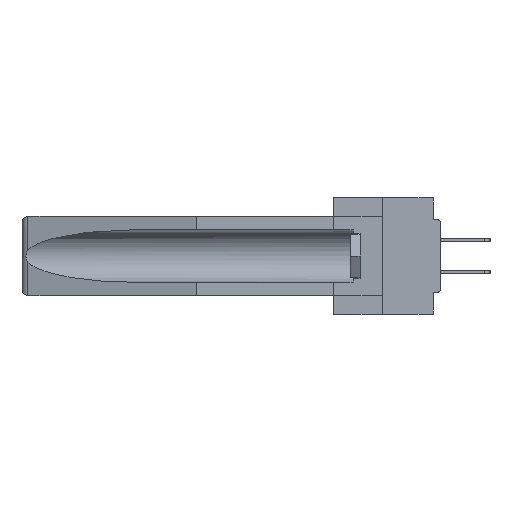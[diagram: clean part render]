
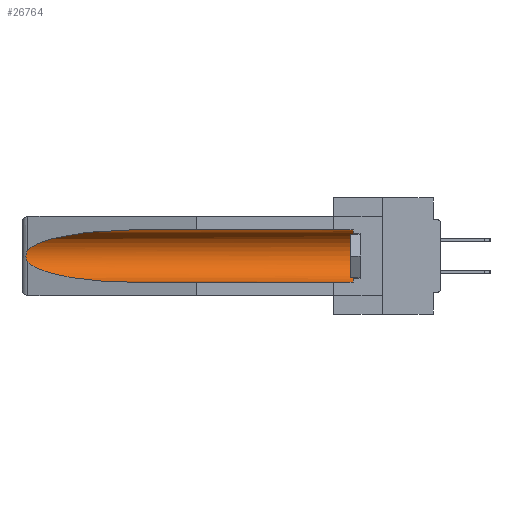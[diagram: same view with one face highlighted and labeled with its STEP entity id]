
A CAD part, left-side view. The second image highlights one B-rep face of the part: STEP entity #26764.
In plain terms, the highlighted cylindrical face has radius 2.857 mm (diameter 5.715 mm), a partial arc.
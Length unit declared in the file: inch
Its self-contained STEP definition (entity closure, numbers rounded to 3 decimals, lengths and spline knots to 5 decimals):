
#1391 = DIRECTION ( 'NONE',  ( 0., -1., 0. ) ) ;
#2315 = CARTESIAN_POINT ( 'NONE',  ( 0.26537, 1.52718, -0.14972 ) ) ;
#2496 = CARTESIAN_POINT ( 'NONE',  ( 0.155, 1.07973, -0.284 ) ) ;
#2711 = CARTESIAN_POINT ( 'NONE',  ( 0.26655, 1.53094, -0.18657 ) ) ;
#2994 = CARTESIAN_POINT ( 'NONE',  ( 0.155, -0.30754, -0.284 ) ) ;
#4425 = ORIENTED_EDGE ( 'NONE', *, *, #5742, .T. ) ;
#5557 = CARTESIAN_POINT ( 'NONE',  ( 0.155, -0.30754, -0.059 ) ) ;
#5742 = EDGE_CURVE ( 'NONE', #29411, #37404, #18426, .T. ) ;
#5941 = AXIS2_PLACEMENT_3D ( 'NONE', #20627, #11267, #35576 ) ;
#6020 = ORIENTED_EDGE ( 'NONE', *, *, #9416, .T. ) ;
#6923 = EDGE_CURVE ( 'NONE', #13804, #29556, #30846, .T. ) ;
#6948 = LINE ( 'NONE', #5557, #38932 ) ;
#7274 = VECTOR ( 'NONE', #39715, 39.37008 ) ;
#8027 = EDGE_LOOP ( 'NONE', ( #38300, #6020, #4425, #25657, #29687, #33324 ) ) ;
#8383 = CARTESIAN_POINT ( 'NONE',  ( 0.155, 1.07973, -0.284 ) ) ;
#8707 = DIRECTION ( 'NONE',  ( 0., 1., 0. ) ) ;
#9004 = VERTEX_POINT ( 'NONE', #38058 ) ;
#9416 = EDGE_CURVE ( 'NONE', #30108, #29411, #28634, .T. ) ;
#11267 = DIRECTION ( 'NONE',  ( 0., 1., 0. ) ) ;
#12777 = CARTESIAN_POINT ( 'NONE',  ( 0.26537, 1.52718, -0.14972 ) ) ;
#13077 = EDGE_CURVE ( 'NONE', #29556, #9004, #6948, .T. ) ;
#13804 = VERTEX_POINT ( 'NONE', #23832 ) ;
#14434 = CARTESIAN_POINT ( 'NONE',  ( 0.26537, 1.52718, -0.19328 ) ) ;
#14963 = EDGE_CURVE ( 'NONE', #9004, #30108, #29880, .T. ) ;
#16250 = CARTESIAN_POINT ( 'NONE',  ( 0.2675, 1.53308, -0.17534 ) ) ;
#16703 = CARTESIAN_POINT ( 'NONE',  ( 0.155, 0.126, -0.1715 ) ) ;
#18426 =( BOUNDED_CURVE ( )  B_SPLINE_CURVE ( 3, ( #14434, #21059, #36138, #2496 ),
 .UNSPECIFIED., .F., .F. ) 
 B_SPLINE_CURVE_WITH_KNOTS ( ( 4, 4 ),
 ( 0.1948, 1.5708 ),
 .UNSPECIFIED. ) 
 CURVE ( )  GEOMETRIC_REPRESENTATION_ITEM ( )  RATIONAL_B_SPLINE_CURVE ( ( 1., 0.848, 0.848, 1. ) ) 
 REPRESENTATION_ITEM ( '' )  );
#18879 = CARTESIAN_POINT ( 'NONE',  ( 0.155, 1.07973, -0.059 ) ) ;
#20627 = CARTESIAN_POINT ( 'NONE',  ( 0.155, -0.30754, -0.1715 ) ) ;
#20876 = CARTESIAN_POINT ( 'NONE',  ( 0.2673, 1.53269, -0.17917 ) ) ;
#21059 = CARTESIAN_POINT ( 'NONE',  ( 0.25451, 1.48313, -0.24835 ) ) ;
#21578 = CARTESIAN_POINT ( 'NONE',  ( 0.21114, 1.30732, -0.059 ) ) ;
#21635 = CARTESIAN_POINT ( 'NONE',  ( 0.26537, 1.52718, -0.19328 ) ) ;
#21881 = CARTESIAN_POINT ( 'NONE',  ( 0.2673, 1.5327, -0.16383 ) ) ;
#22478 = CARTESIAN_POINT ( 'NONE',  ( 0.26537, 1.52718, -0.14972 ) ) ;
#22565 = CARTESIAN_POINT ( 'NONE',  ( 0.2675, 1.53308, -0.16763 ) ) ;
#23373 = CARTESIAN_POINT ( 'NONE',  ( 0.155, 0.126, -0.059 ) ) ;
#23832 = CARTESIAN_POINT ( 'NONE',  ( 0.155, 0.126, -0.284 ) ) ;
#24254 = FACE_OUTER_BOUND ( 'NONE', #8027, .T. ) ;
#25354 = AXIS2_PLACEMENT_3D ( 'NONE', #16703, #1391, #28897 ) ;
#25657 = ORIENTED_EDGE ( 'NONE', *, *, #28810, .F. ) ;
#26764 = ADVANCED_FACE ( 'NONE', ( #24254 ), #35944, .F. ) ;
#28634 = B_SPLINE_CURVE_WITH_KNOTS ( 'NONE', 3,
 ( #22478, #34951, #37507, #21881, #22565, #16250, #20876, #2711, #36692, #38647 ),
 .UNSPECIFIED., .F., .F.,
 ( 4, 2, 2, 2, 4 ),
 ( 0., 0.00029, 0.00058, 0.00087, 0.00117 ),
 .UNSPECIFIED. ) ;
#28810 = EDGE_CURVE ( 'NONE', #13804, #37404, #33936, .T. ) ;
#28897 = DIRECTION ( 'NONE',  ( 0., 0., 1. ) ) ;
#29411 = VERTEX_POINT ( 'NONE', #21635 ) ;
#29556 = VERTEX_POINT ( 'NONE', #23373 ) ;
#29687 = ORIENTED_EDGE ( 'NONE', *, *, #6923, .T. ) ;
#29880 =( BOUNDED_CURVE ( )  B_SPLINE_CURVE ( 3, ( #18879, #21578, #34192, #12777 ),
 .UNSPECIFIED., .F., .F. ) 
 B_SPLINE_CURVE_WITH_KNOTS ( ( 4, 4 ),
 ( 4.71239, 6.08839 ),
 .UNSPECIFIED. ) 
 CURVE ( )  GEOMETRIC_REPRESENTATION_ITEM ( )  RATIONAL_B_SPLINE_CURVE ( ( 1., 0.848, 0.848, 1. ) ) 
 REPRESENTATION_ITEM ( '' )  );
#30108 = VERTEX_POINT ( 'NONE', #2315 ) ;
#30846 = CIRCLE ( 'NONE', #25354, 0.1125 ) ;
#33324 = ORIENTED_EDGE ( 'NONE', *, *, #13077, .T. ) ;
#33936 = LINE ( 'NONE', #2994, #7274 ) ;
#34192 = CARTESIAN_POINT ( 'NONE',  ( 0.25451, 1.48313, -0.09465 ) ) ;
#34951 = CARTESIAN_POINT ( 'NONE',  ( 0.26597, 1.52961, -0.15275 ) ) ;
#35576 = DIRECTION ( 'NONE',  ( 0., 0., 1. ) ) ;
#35944 = CYLINDRICAL_SURFACE ( 'NONE', #5941, 0.1125 ) ;
#36138 = CARTESIAN_POINT ( 'NONE',  ( 0.21114, 1.30732, -0.284 ) ) ;
#36692 = CARTESIAN_POINT ( 'NONE',  ( 0.26597, 1.5296, -0.19026 ) ) ;
#37404 = VERTEX_POINT ( 'NONE', #8383 ) ;
#37507 = CARTESIAN_POINT ( 'NONE',  ( 0.26654, 1.53092, -0.15636 ) ) ;
#38058 = CARTESIAN_POINT ( 'NONE',  ( 0.155, 1.07973, -0.059 ) ) ;
#38300 = ORIENTED_EDGE ( 'NONE', *, *, #14963, .T. ) ;
#38647 = CARTESIAN_POINT ( 'NONE',  ( 0.26537, 1.52718, -0.19328 ) ) ;
#38932 = VECTOR ( 'NONE', #8707, 39.37008 ) ;
#39715 = DIRECTION ( 'NONE',  ( 0., 1., 0. ) ) ;
